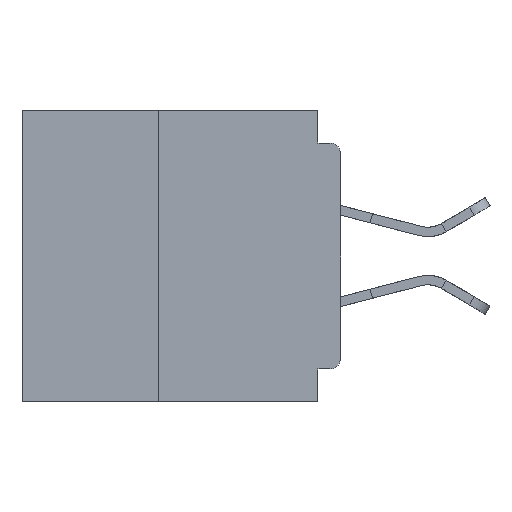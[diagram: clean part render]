
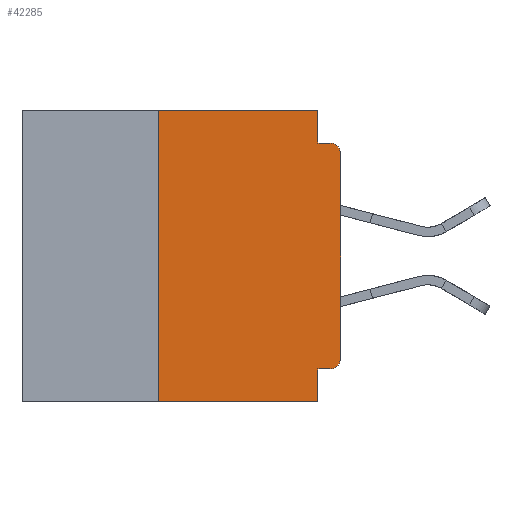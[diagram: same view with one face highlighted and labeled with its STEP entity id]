
A CAD part, left-side view. The second image highlights one B-rep face of the part: STEP entity #42285.
In plain terms, the highlighted planar face has unit normal (-1, 0, 0).
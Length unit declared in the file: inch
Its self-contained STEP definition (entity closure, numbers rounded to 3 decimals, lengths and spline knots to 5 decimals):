
#52 = VERTEX_POINT ( 'NONE', #36213 ) ;
#518 = ORIENTED_EDGE ( 'NONE', *, *, #30018, .T. ) ;
#618 = EDGE_CURVE ( 'NONE', #12221, #40707, #16500, .T. ) ;
#1372 = EDGE_CURVE ( 'NONE', #39215, #52, #38336, .T. ) ;
#2028 = CARTESIAN_POINT ( 'NONE',  ( 0., 0.437, -0.4 ) ) ;
#2375 = VECTOR ( 'NONE', #8107, 39.37008 ) ;
#2513 = CARTESIAN_POINT ( 'NONE',  ( 0., 0.437, 0. ) ) ;
#2762 = CARTESIAN_POINT ( 'NONE',  ( 0., 0.031, -0.4 ) ) ;
#2775 = DIRECTION ( 'NONE',  ( 0., 0., -1. ) ) ;
#3539 = EDGE_LOOP ( 'NONE', ( #518, #33632, #14475, #18132, #48400, #12676, #45489, #24783, #24653, #15697 ) ) ;
#4114 = CARTESIAN_POINT ( 'NONE',  ( 0., 0.437, 0. ) ) ;
#5908 = EDGE_CURVE ( 'NONE', #49123, #39215, #20068, .T. ) ;
#5937 = DIRECTION ( 'NONE',  ( 0., -1., 0. ) ) ;
#6053 = AXIS2_PLACEMENT_3D ( 'NONE', #37745, #14879, #41554 ) ;
#6656 = CIRCLE ( 'NONE', #22240, 0.015 ) ;
#7175 = LINE ( 'NONE', #2028, #26459 ) ;
#7770 = CARTESIAN_POINT ( 'NONE',  ( 0., 0.015, -0.045 ) ) ;
#7772 = CARTESIAN_POINT ( 'NONE',  ( 0., 0.25, -0.4 ) ) ;
#8107 = DIRECTION ( 'NONE',  ( 0., -1., 0. ) ) ;
#9949 = CARTESIAN_POINT ( 'NONE',  ( 0., 0.031, -0.355 ) ) ;
#12221 = VERTEX_POINT ( 'NONE', #9949 ) ;
#12676 = ORIENTED_EDGE ( 'NONE', *, *, #5908, .F. ) ;
#12721 = LINE ( 'NONE', #31791, #19358 ) ;
#13703 = CARTESIAN_POINT ( 'NONE',  ( 0., 0., -0.355 ) ) ;
#14475 = ORIENTED_EDGE ( 'NONE', *, *, #19899, .F. ) ;
#14879 = DIRECTION ( 'NONE',  ( -1., 0., 0. ) ) ;
#15697 = ORIENTED_EDGE ( 'NONE', *, *, #21034, .T. ) ;
#15795 = DIRECTION ( 'NONE',  ( 0., 0., 1. ) ) ;
#16500 = LINE ( 'NONE', #2762, #35630 ) ;
#18132 = ORIENTED_EDGE ( 'NONE', *, *, #47357, .F. ) ;
#19082 = AXIS2_PLACEMENT_3D ( 'NONE', #4114, #42434, #19665 ) ;
#19268 = VECTOR ( 'NONE', #37043, 39.37008 ) ;
#19358 = VECTOR ( 'NONE', #35628, 39.37008 ) ;
#19665 = DIRECTION ( 'NONE',  ( 0., 0., -1. ) ) ;
#19854 = VERTEX_POINT ( 'NONE', #7770 ) ;
#19899 = EDGE_CURVE ( 'NONE', #38522, #19854, #43139, .T. ) ;
#20068 = LINE ( 'NONE', #38808, #28997 ) ;
#21034 = EDGE_CURVE ( 'NONE', #43436, #24498, #22882, .T. ) ;
#21171 = DIRECTION ( 'NONE',  ( -1., 0., 0. ) ) ;
#21735 = VECTOR ( 'NONE', #44246, 39.37008 ) ;
#22066 = VECTOR ( 'NONE', #42415, 39.37008 ) ;
#22240 = AXIS2_PLACEMENT_3D ( 'NONE', #43950, #21171, #47727 ) ;
#22882 = CIRCLE ( 'NONE', #6053, 0.015 ) ;
#22956 = CARTESIAN_POINT ( 'NONE',  ( 0., 0.031, -0.045 ) ) ;
#23223 = CARTESIAN_POINT ( 'NONE',  ( 0., 0.25, 0. ) ) ;
#23271 = LINE ( 'NONE', #38622, #22066 ) ;
#24498 = VERTEX_POINT ( 'NONE', #45192 ) ;
#24653 = ORIENTED_EDGE ( 'NONE', *, *, #42583, .F. ) ;
#24783 = ORIENTED_EDGE ( 'NONE', *, *, #618, .F. ) ;
#26459 = VECTOR ( 'NONE', #5937, 39.37008 ) ;
#26593 = EDGE_CURVE ( 'NONE', #44367, #19854, #6656, .T. ) ;
#27243 = EDGE_CURVE ( 'NONE', #49123, #40707, #7175, .T. ) ;
#28997 = VECTOR ( 'NONE', #15795, 39.37008 ) ;
#30018 = EDGE_CURVE ( 'NONE', #24498, #44367, #23271, .T. ) ;
#31791 = CARTESIAN_POINT ( 'NONE',  ( 0., 0.031, 0. ) ) ;
#31884 = LINE ( 'NONE', #13703, #21735 ) ;
#33632 = ORIENTED_EDGE ( 'NONE', *, *, #26593, .T. ) ;
#35628 = DIRECTION ( 'NONE',  ( 0., 0., -1. ) ) ;
#35630 = VECTOR ( 'NONE', #2775, 39.37008 ) ;
#36213 = CARTESIAN_POINT ( 'NONE',  ( 0., 0.031, 0. ) ) ;
#37043 = DIRECTION ( 'NONE',  ( 0., -1., 0. ) ) ;
#37247 = FACE_OUTER_BOUND ( 'NONE', #3539, .T. ) ;
#37745 = CARTESIAN_POINT ( 'NONE',  ( 0., 0.015, -0.34 ) ) ;
#38336 = LINE ( 'NONE', #2513, #19268 ) ;
#38522 = VERTEX_POINT ( 'NONE', #22956 ) ;
#38622 = CARTESIAN_POINT ( 'NONE',  ( 0., 0., 0. ) ) ;
#38808 = CARTESIAN_POINT ( 'NONE',  ( 0., 0.25, -0.4 ) ) ;
#39215 = VERTEX_POINT ( 'NONE', #23223 ) ;
#40707 = VERTEX_POINT ( 'NONE', #47287 ) ;
#41554 = DIRECTION ( 'NONE',  ( 0., 0., -1. ) ) ;
#41938 = CARTESIAN_POINT ( 'NONE',  ( 0., 0., -0.06 ) ) ;
#42276 = PLANE ( 'NONE',  #19082 ) ;
#42285 = ADVANCED_FACE ( 'NONE', ( #37247 ), #42276, .F. ) ;
#42415 = DIRECTION ( 'NONE',  ( 0., 0., 1. ) ) ;
#42434 = DIRECTION ( 'NONE',  ( 1., 0., 0. ) ) ;
#42583 = EDGE_CURVE ( 'NONE', #43436, #12221, #31884, .T. ) ;
#43139 = LINE ( 'NONE', #46311, #2375 ) ;
#43436 = VERTEX_POINT ( 'NONE', #45623 ) ;
#43950 = CARTESIAN_POINT ( 'NONE',  ( 0., 0.015, -0.06 ) ) ;
#44246 = DIRECTION ( 'NONE',  ( 0., 1., 0. ) ) ;
#44367 = VERTEX_POINT ( 'NONE', #41938 ) ;
#45192 = CARTESIAN_POINT ( 'NONE',  ( 0., 0., -0.34 ) ) ;
#45489 = ORIENTED_EDGE ( 'NONE', *, *, #27243, .T. ) ;
#45623 = CARTESIAN_POINT ( 'NONE',  ( 0., 0.015, -0.355 ) ) ;
#46311 = CARTESIAN_POINT ( 'NONE',  ( 0., 0., -0.045 ) ) ;
#47287 = CARTESIAN_POINT ( 'NONE',  ( 0., 0.031, -0.4 ) ) ;
#47357 = EDGE_CURVE ( 'NONE', #52, #38522, #12721, .T. ) ;
#47727 = DIRECTION ( 'NONE',  ( 0., 0., -1. ) ) ;
#48400 = ORIENTED_EDGE ( 'NONE', *, *, #1372, .F. ) ;
#49123 = VERTEX_POINT ( 'NONE', #7772 ) ;
